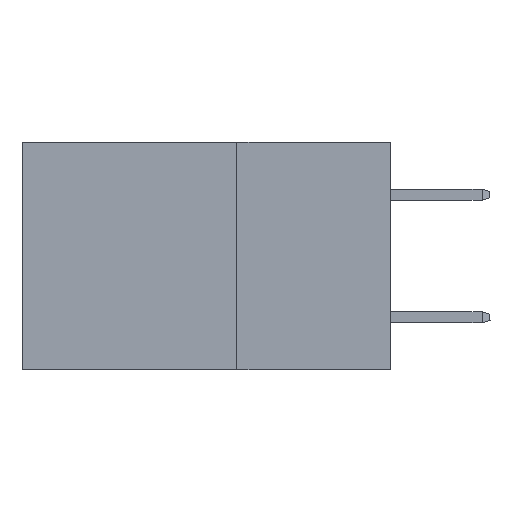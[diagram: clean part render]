
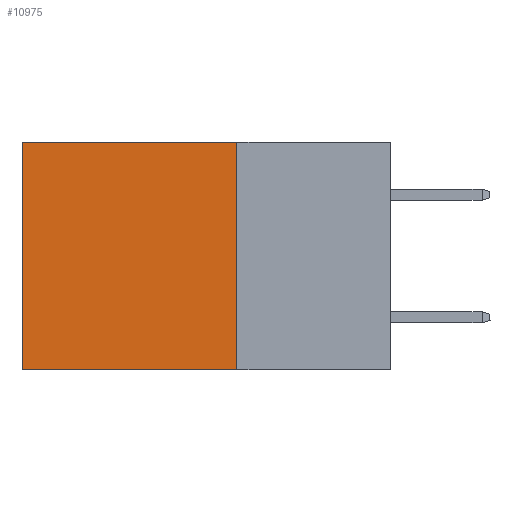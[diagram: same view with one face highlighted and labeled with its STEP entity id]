
A CAD part, left-side view. The second image highlights one B-rep face of the part: STEP entity #10975.
In plain terms, the highlighted planar face has unit normal (-1, 0, 0).
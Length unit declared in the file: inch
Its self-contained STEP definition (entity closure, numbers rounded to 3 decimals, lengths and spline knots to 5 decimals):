
#448 = ORIENTED_EDGE ( 'NONE', *, *, #1723, .F. ) ;
#648 = CARTESIAN_POINT ( 'NONE',  ( 0.2875, 0.6, 0. ) ) ;
#1723 = EDGE_CURVE ( 'NONE', #17554, #13886, #27892, .T. ) ;
#2021 = PLANE ( 'NONE',  #28562 ) ;
#2606 = CARTESIAN_POINT ( 'NONE',  ( 0.2875, 0.25, 0. ) ) ;
#4175 = VECTOR ( 'NONE', #12026, 39.37008 ) ;
#4369 = LINE ( 'NONE', #29074, #24844 ) ;
#4403 = ORIENTED_EDGE ( 'NONE', *, *, #27985, .T. ) ;
#4958 = EDGE_LOOP ( 'NONE', ( #8666, #19274, #448, #4403 ) ) ;
#6970 = LINE ( 'NONE', #648, #8940 ) ;
#7554 = CARTESIAN_POINT ( 'NONE',  ( 0.2875, 0.25, 0. ) ) ;
#8201 = LINE ( 'NONE', #8508, #23455 ) ;
#8488 = DIRECTION ( 'NONE',  ( 1., 0., 0. ) ) ;
#8508 = CARTESIAN_POINT ( 'NONE',  ( 0.2875, 0.25, 0. ) ) ;
#8666 = ORIENTED_EDGE ( 'NONE', *, *, #19633, .T. ) ;
#8940 = VECTOR ( 'NONE', #13979, 39.37008 ) ;
#9559 = CARTESIAN_POINT ( 'NONE',  ( 0.2875, 0.25, -0.37 ) ) ;
#10820 = DIRECTION ( 'NONE',  ( 0., 1., 0. ) ) ;
#10975 = ADVANCED_FACE ( 'NONE', ( #13394 ), #2021, .F. ) ;
#11121 = CARTESIAN_POINT ( 'NONE',  ( 0.2875, 0.6, 0. ) ) ;
#11161 = CARTESIAN_POINT ( 'NONE',  ( 0.2875, 0.25, 0. ) ) ;
#12026 = DIRECTION ( 'NONE',  ( 0., 0., -1. ) ) ;
#13394 = FACE_OUTER_BOUND ( 'NONE', #4958, .T. ) ;
#13886 = VERTEX_POINT ( 'NONE', #9559 ) ;
#13979 = DIRECTION ( 'NONE',  ( 0., 0., -1. ) ) ;
#17319 = DIRECTION ( 'NONE',  ( 0., 1., 0. ) ) ;
#17554 = VERTEX_POINT ( 'NONE', #2606 ) ;
#18435 = CARTESIAN_POINT ( 'NONE',  ( 0.2875, 0.6, -0.37 ) ) ;
#19274 = ORIENTED_EDGE ( 'NONE', *, *, #25207, .F. ) ;
#19633 = EDGE_CURVE ( 'NONE', #19958, #20118, #6970, .T. ) ;
#19958 = VERTEX_POINT ( 'NONE', #11121 ) ;
#20118 = VERTEX_POINT ( 'NONE', #18435 ) ;
#20288 = DIRECTION ( 'NONE',  ( 0., 0., -1. ) ) ;
#23455 = VECTOR ( 'NONE', #17319, 39.37008 ) ;
#24844 = VECTOR ( 'NONE', #10820, 39.37008 ) ;
#25207 = EDGE_CURVE ( 'NONE', #13886, #20118, #4369, .T. ) ;
#27892 = LINE ( 'NONE', #7554, #4175 ) ;
#27985 = EDGE_CURVE ( 'NONE', #17554, #19958, #8201, .T. ) ;
#28562 = AXIS2_PLACEMENT_3D ( 'NONE', #11161, #8488, #20288 ) ;
#29074 = CARTESIAN_POINT ( 'NONE',  ( 0.2875, 0.25, -0.37 ) ) ;
